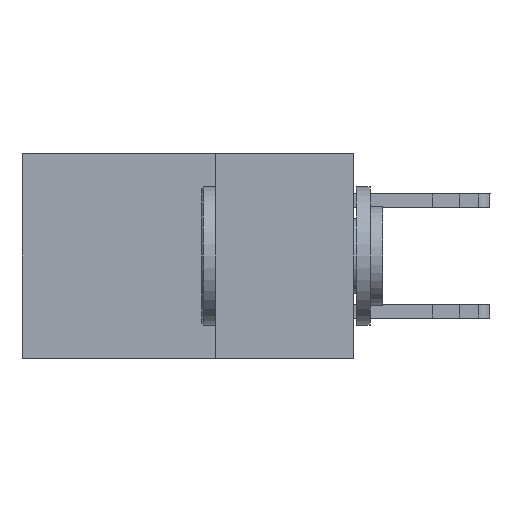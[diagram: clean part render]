
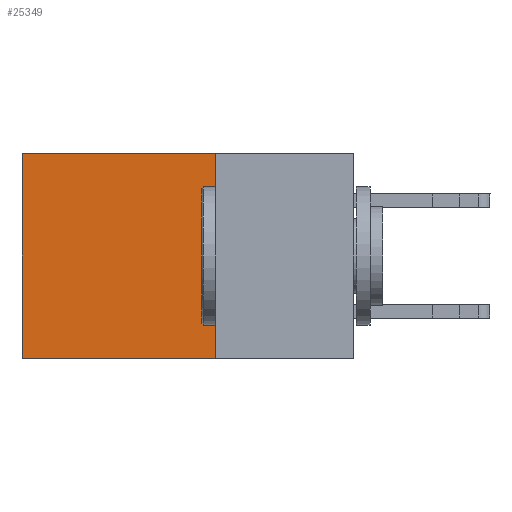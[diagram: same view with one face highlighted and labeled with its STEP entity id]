
A CAD part, left-side view. The second image highlights one B-rep face of the part: STEP entity #25349.
In plain terms, the highlighted planar face has unit normal (-1, 0, 0).
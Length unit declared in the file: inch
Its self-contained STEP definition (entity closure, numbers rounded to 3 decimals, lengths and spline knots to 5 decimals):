
#249 = VECTOR ( 'NONE', #26052, 39.37008 ) ;
#337 = VECTOR ( 'NONE', #19183, 39.37008 ) ;
#1234 = LINE ( 'NONE', #22595, #5269 ) ;
#1394 = CARTESIAN_POINT ( 'NONE',  ( 0.2875, 0.25, 0. ) ) ;
#4118 = LINE ( 'NONE', #11958, #26316 ) ;
#4240 = EDGE_CURVE ( 'NONE', #30608, #21878, #1234, .T. ) ;
#5269 = VECTOR ( 'NONE', #12789, 39.37008 ) ;
#5432 = EDGE_CURVE ( 'NONE', #30342, #30608, #7228, .T. ) ;
#6913 = VERTEX_POINT ( 'NONE', #26152 ) ;
#7228 = LINE ( 'NONE', #1394, #337 ) ;
#7430 = PLANE ( 'NONE',  #17953 ) ;
#8739 = ORIENTED_EDGE ( 'NONE', *, *, #20112, .F. ) ;
#10033 = DIRECTION ( 'NONE',  ( 0., 0., -1. ) ) ;
#11958 = CARTESIAN_POINT ( 'NONE',  ( 0.2875, 0.25, -0.37 ) ) ;
#12494 = FACE_OUTER_BOUND ( 'NONE', #28967, .T. ) ;
#12501 = CARTESIAN_POINT ( 'NONE',  ( 0.2875, 0.25, 0. ) ) ;
#12789 = DIRECTION ( 'NONE',  ( 0., 0., -1. ) ) ;
#13823 = CARTESIAN_POINT ( 'NONE',  ( 0.2875, 0.6, 0. ) ) ;
#17953 = AXIS2_PLACEMENT_3D ( 'NONE', #12501, #30445, #10033 ) ;
#19183 = DIRECTION ( 'NONE',  ( 0., 1., 0. ) ) ;
#19633 = DIRECTION ( 'NONE',  ( 0., 1., 0. ) ) ;
#20112 = EDGE_CURVE ( 'NONE', #30342, #6913, #28450, .T. ) ;
#20604 = ORIENTED_EDGE ( 'NONE', *, *, #25508, .F. ) ;
#21863 = ORIENTED_EDGE ( 'NONE', *, *, #4240, .T. ) ;
#21878 = VERTEX_POINT ( 'NONE', #30642 ) ;
#22595 = CARTESIAN_POINT ( 'NONE',  ( 0.2875, 0.6, 0. ) ) ;
#22702 = CARTESIAN_POINT ( 'NONE',  ( 0.2875, 0.25, 0. ) ) ;
#25349 = ADVANCED_FACE ( 'NONE', ( #12494 ), #7430, .F. ) ;
#25508 = EDGE_CURVE ( 'NONE', #6913, #21878, #4118, .T. ) ;
#26052 = DIRECTION ( 'NONE',  ( 0., 0., -1. ) ) ;
#26152 = CARTESIAN_POINT ( 'NONE',  ( 0.2875, 0.25, -0.37 ) ) ;
#26316 = VECTOR ( 'NONE', #19633, 39.37008 ) ;
#28096 = CARTESIAN_POINT ( 'NONE',  ( 0.2875, 0.25, 0. ) ) ;
#28450 = LINE ( 'NONE', #28096, #249 ) ;
#28967 = EDGE_LOOP ( 'NONE', ( #21863, #20604, #8739, #30917 ) ) ;
#30342 = VERTEX_POINT ( 'NONE', #22702 ) ;
#30445 = DIRECTION ( 'NONE',  ( 1., 0., 0. ) ) ;
#30608 = VERTEX_POINT ( 'NONE', #13823 ) ;
#30642 = CARTESIAN_POINT ( 'NONE',  ( 0.2875, 0.6, -0.37 ) ) ;
#30917 = ORIENTED_EDGE ( 'NONE', *, *, #5432, .T. ) ;
